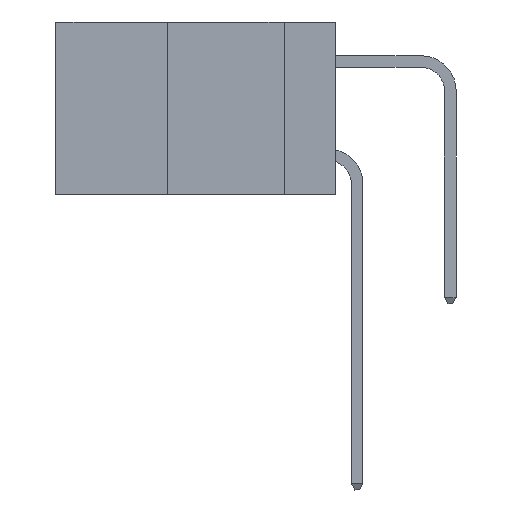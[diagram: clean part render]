
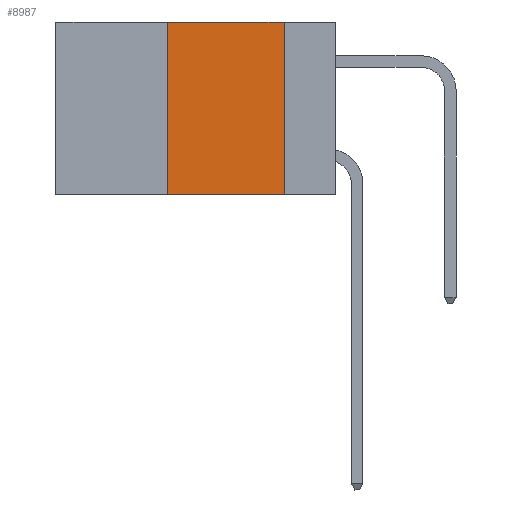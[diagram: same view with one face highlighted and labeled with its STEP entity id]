
A CAD part, left-side view. The second image highlights one B-rep face of the part: STEP entity #8987.
In plain terms, the highlighted planar face has unit normal (-1, 0, 0).
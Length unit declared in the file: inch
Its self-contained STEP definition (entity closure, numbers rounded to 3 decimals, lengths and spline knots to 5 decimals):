
#138 = CARTESIAN_POINT ( 'NONE',  ( 0., 0.11, 0. ) ) ;
#145 = CARTESIAN_POINT ( 'NONE',  ( 0., 0.36, 0. ) ) ;
#343 = CARTESIAN_POINT ( 'NONE',  ( 0., 0.6, -0.37 ) ) ;
#351 = VECTOR ( 'NONE', #18170, 39.37008 ) ;
#405 = VERTEX_POINT ( 'NONE', #17397 ) ;
#652 = VERTEX_POINT ( 'NONE', #15114 ) ;
#1090 = DIRECTION ( 'NONE',  ( 0., 0., -1. ) ) ;
#1724 = LINE ( 'NONE', #343, #21106 ) ;
#3233 = VECTOR ( 'NONE', #13129, 39.37008 ) ;
#3764 = EDGE_CURVE ( 'NONE', #27263, #652, #8755, .T. ) ;
#3950 = EDGE_CURVE ( 'NONE', #405, #27263, #8047, .T. ) ;
#4945 = FACE_OUTER_BOUND ( 'NONE', #7554, .T. ) ;
#7098 = EDGE_CURVE ( 'NONE', #11510, #652, #1724, .T. ) ;
#7554 = EDGE_LOOP ( 'NONE', ( #22308, #21854, #16167, #21255 ) ) ;
#7613 = CARTESIAN_POINT ( 'NONE',  ( 0., 0.11, 0. ) ) ;
#8047 = LINE ( 'NONE', #12965, #21728 ) ;
#8755 = LINE ( 'NONE', #7613, #351 ) ;
#8987 = ADVANCED_FACE ( 'NONE', ( #4945 ), #9723, .F. ) ;
#9723 = PLANE ( 'NONE',  #18025 ) ;
#10655 = DIRECTION ( 'NONE',  ( 0., -1., 0. ) ) ;
#11510 = VERTEX_POINT ( 'NONE', #27149 ) ;
#12690 = DIRECTION ( 'NONE',  ( 0., -1., 0. ) ) ;
#12965 = CARTESIAN_POINT ( 'NONE',  ( 0., 0.6, 0. ) ) ;
#13129 = DIRECTION ( 'NONE',  ( 0., 0., 1. ) ) ;
#13715 = CARTESIAN_POINT ( 'NONE',  ( 0., 0.6, 0. ) ) ;
#13891 = DIRECTION ( 'NONE',  ( 1., 0., 0. ) ) ;
#15114 = CARTESIAN_POINT ( 'NONE',  ( 0., 0.11, -0.37 ) ) ;
#16167 = ORIENTED_EDGE ( 'NONE', *, *, #23718, .F. ) ;
#17397 = CARTESIAN_POINT ( 'NONE',  ( 0., 0.36, 0. ) ) ;
#18025 = AXIS2_PLACEMENT_3D ( 'NONE', #13715, #13891, #1090 ) ;
#18170 = DIRECTION ( 'NONE',  ( 0., 0., -1. ) ) ;
#20271 = LINE ( 'NONE', #145, #3233 ) ;
#21106 = VECTOR ( 'NONE', #12690, 39.37008 ) ;
#21255 = ORIENTED_EDGE ( 'NONE', *, *, #7098, .T. ) ;
#21728 = VECTOR ( 'NONE', #10655, 39.37008 ) ;
#21854 = ORIENTED_EDGE ( 'NONE', *, *, #3950, .F. ) ;
#22308 = ORIENTED_EDGE ( 'NONE', *, *, #3764, .F. ) ;
#23718 = EDGE_CURVE ( 'NONE', #11510, #405, #20271, .T. ) ;
#27149 = CARTESIAN_POINT ( 'NONE',  ( 0., 0.36, -0.37 ) ) ;
#27263 = VERTEX_POINT ( 'NONE', #138 ) ;
